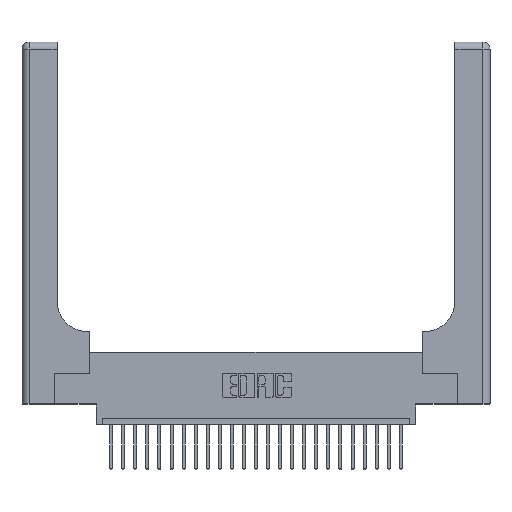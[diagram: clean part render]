
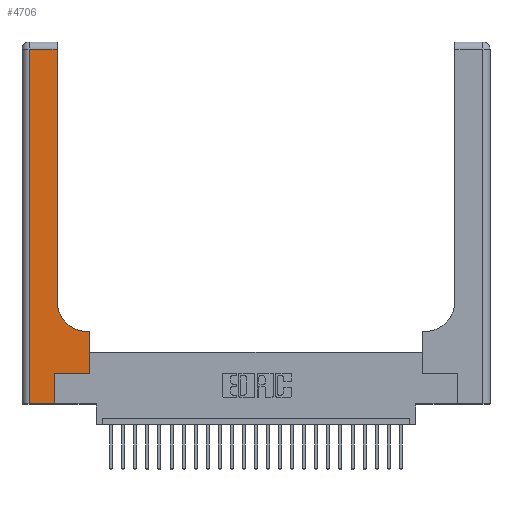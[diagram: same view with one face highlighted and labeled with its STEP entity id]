
A CAD part, top view. The second image highlights one B-rep face of the part: STEP entity #4706.
In plain terms, the highlighted planar face has unit normal (0, 0, 1).
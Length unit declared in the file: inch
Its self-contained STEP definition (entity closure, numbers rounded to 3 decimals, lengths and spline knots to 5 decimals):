
#183 = VERTEX_POINT ( 'NONE', #3995 ) ;
#387 = LINE ( 'NONE', #11494, #11585 ) ;
#464 = CARTESIAN_POINT ( 'NONE',  ( 0.06, 0., 0.37 ) ) ;
#2063 = VERTEX_POINT ( 'NONE', #16297 ) ;
#2518 = VERTEX_POINT ( 'NONE', #10195 ) ;
#2962 = EDGE_CURVE ( 'NONE', #2063, #18216, #387, .T. ) ;
#3097 = VERTEX_POINT ( 'NONE', #15822 ) ;
#3435 = VECTOR ( 'NONE', #18888, 39.37008 ) ;
#3995 = CARTESIAN_POINT ( 'NONE',  ( 0.269, 0., 0.37 ) ) ;
#4355 = DIRECTION ( 'NONE',  ( -1., 0., 0. ) ) ;
#4496 = CARTESIAN_POINT ( 'NONE',  ( 0., 2.94, 0.37 ) ) ;
#4638 = ORIENTED_EDGE ( 'NONE', *, *, #6326, .T. ) ;
#4706 = ADVANCED_FACE ( 'NONE', ( #14672 ), #10578, .F. ) ;
#5338 = EDGE_CURVE ( 'NONE', #3097, #17423, #24492, .T. ) ;
#5381 = VERTEX_POINT ( 'NONE', #20317 ) ;
#5893 = CARTESIAN_POINT ( 'NONE',  ( 0.2915, 3., 0.37 ) ) ;
#6193 = DIRECTION ( 'NONE',  ( 0., 0., -1. ) ) ;
#6215 = CARTESIAN_POINT ( 'NONE',  ( 0., 3., 0.37 ) ) ;
#6326 = EDGE_CURVE ( 'NONE', #17423, #2518, #12043, .T. ) ;
#6481 = AXIS2_PLACEMENT_3D ( 'NONE', #6215, #12258, #4355 ) ;
#7183 = AXIS2_PLACEMENT_3D ( 'NONE', #7898, #6193, #14195 ) ;
#7255 = DIRECTION ( 'NONE',  ( 0., 1., 0. ) ) ;
#7308 = LINE ( 'NONE', #21157, #21604 ) ;
#7898 = CARTESIAN_POINT ( 'NONE',  ( 0.5415, 0.85, 0.37 ) ) ;
#7949 = LINE ( 'NONE', #4496, #3435 ) ;
#9947 = ORIENTED_EDGE ( 'NONE', *, *, #5338, .T. ) ;
#10195 = CARTESIAN_POINT ( 'NONE',  ( 0.2915, 2.94, 0.37 ) ) ;
#10371 = CARTESIAN_POINT ( 'NONE',  ( 0.2915, 0.85, 0.37 ) ) ;
#10549 = EDGE_LOOP ( 'NONE', ( #4638, #14538, #17648, #22943, #21397, #15918, #17096, #17260, #9947 ) ) ;
#10578 = PLANE ( 'NONE',  #6481 ) ;
#11047 = DIRECTION ( 'NONE',  ( 0., 1., 0. ) ) ;
#11396 = DIRECTION ( 'NONE',  ( 1., 0., 0. ) ) ;
#11494 = CARTESIAN_POINT ( 'NONE',  ( 0.06, 3., 0.37 ) ) ;
#11503 = EDGE_CURVE ( 'NONE', #15207, #18057, #20332, .T. ) ;
#11585 = VECTOR ( 'NONE', #23476, 39.37008 ) ;
#11770 = DIRECTION ( 'NONE',  ( 0., 1., 0. ) ) ;
#11850 = VECTOR ( 'NONE', #11920, 39.37008 ) ;
#11920 = DIRECTION ( 'NONE',  ( 1., 0., 0. ) ) ;
#12043 = LINE ( 'NONE', #5893, #26055 ) ;
#12258 = DIRECTION ( 'NONE',  ( 0., 0., -1. ) ) ;
#13423 = CARTESIAN_POINT ( 'NONE',  ( 0., 0., 0.37 ) ) ;
#13681 = EDGE_CURVE ( 'NONE', #2518, #2063, #7949, .T. ) ;
#13767 = LINE ( 'NONE', #24010, #11850 ) ;
#14005 = CARTESIAN_POINT ( 'NONE',  ( 0.5585, 0.25, 0.37 ) ) ;
#14145 = LINE ( 'NONE', #19340, #21724 ) ;
#14195 = DIRECTION ( 'NONE',  ( 1., 0., 0. ) ) ;
#14538 = ORIENTED_EDGE ( 'NONE', *, *, #13681, .T. ) ;
#14672 = FACE_OUTER_BOUND ( 'NONE', #10549, .T. ) ;
#15207 = VERTEX_POINT ( 'NONE', #16939 ) ;
#15329 = DIRECTION ( 'NONE',  ( -1., 0., 0. ) ) ;
#15822 = CARTESIAN_POINT ( 'NONE',  ( 0.5415, 0.6, 0.37 ) ) ;
#15918 = ORIENTED_EDGE ( 'NONE', *, *, #22678, .T. ) ;
#16297 = CARTESIAN_POINT ( 'NONE',  ( 0.06, 2.94, 0.37 ) ) ;
#16674 = VECTOR ( 'NONE', #11396, 39.37008 ) ;
#16939 = CARTESIAN_POINT ( 'NONE',  ( 0.5585, 0.25, 0.37 ) ) ;
#17096 = ORIENTED_EDGE ( 'NONE', *, *, #11503, .T. ) ;
#17260 = ORIENTED_EDGE ( 'NONE', *, *, #21496, .T. ) ;
#17423 = VERTEX_POINT ( 'NONE', #10371 ) ;
#17483 = VECTOR ( 'NONE', #7255, 39.37008 ) ;
#17648 = ORIENTED_EDGE ( 'NONE', *, *, #2962, .T. ) ;
#17775 = EDGE_CURVE ( 'NONE', #18216, #183, #24007, .T. ) ;
#18057 = VERTEX_POINT ( 'NONE', #22339 ) ;
#18216 = VERTEX_POINT ( 'NONE', #464 ) ;
#18888 = DIRECTION ( 'NONE',  ( -1., 0., 0. ) ) ;
#19340 = CARTESIAN_POINT ( 'NONE',  ( 0.2915, 0.6, 0.37 ) ) ;
#20317 = CARTESIAN_POINT ( 'NONE',  ( 0.269, 0.25, 0.37 ) ) ;
#20332 = LINE ( 'NONE', #14005, #17483 ) ;
#21157 = CARTESIAN_POINT ( 'NONE',  ( 0.269, 0., 0.37 ) ) ;
#21397 = ORIENTED_EDGE ( 'NONE', *, *, #24272, .T. ) ;
#21496 = EDGE_CURVE ( 'NONE', #18057, #3097, #14145, .T. ) ;
#21604 = VECTOR ( 'NONE', #11047, 39.37008 ) ;
#21724 = VECTOR ( 'NONE', #15329, 39.37008 ) ;
#22339 = CARTESIAN_POINT ( 'NONE',  ( 0.5585, 0.6, 0.37 ) ) ;
#22678 = EDGE_CURVE ( 'NONE', #5381, #15207, #13767, .T. ) ;
#22943 = ORIENTED_EDGE ( 'NONE', *, *, #17775, .T. ) ;
#23476 = DIRECTION ( 'NONE',  ( 0., -1., 0. ) ) ;
#24007 = LINE ( 'NONE', #13423, #16674 ) ;
#24010 = CARTESIAN_POINT ( 'NONE',  ( 0.269, 0.25, 0.37 ) ) ;
#24272 = EDGE_CURVE ( 'NONE', #183, #5381, #7308, .T. ) ;
#24492 = CIRCLE ( 'NONE', #7183, 0.25 ) ;
#26055 = VECTOR ( 'NONE', #11770, 39.37008 ) ;
